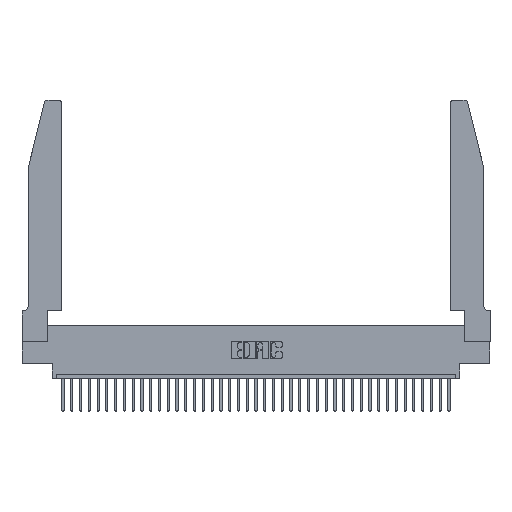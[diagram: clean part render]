
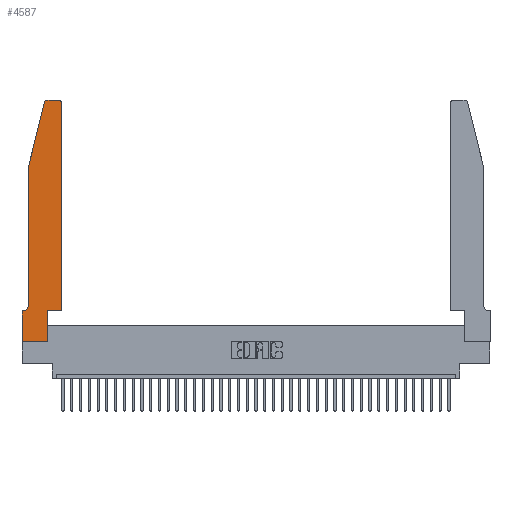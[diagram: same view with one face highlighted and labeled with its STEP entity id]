
A CAD part, top view. The second image highlights one B-rep face of the part: STEP entity #4587.
In plain terms, the highlighted planar face has unit normal (0, 0, 1).
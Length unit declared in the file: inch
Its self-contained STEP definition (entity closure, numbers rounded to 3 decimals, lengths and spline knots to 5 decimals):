
#349 = CARTESIAN_POINT ( 'NONE',  ( 0.284, 2.72, 0.37 ) ) ;
#1829 = AXIS2_PLACEMENT_3D ( 'NONE', #28005, #34072, #10790 ) ;
#2584 = DIRECTION ( 'NONE',  ( 0., 0., 1. ) ) ;
#2587 = AXIS2_PLACEMENT_3D ( 'NONE', #349, #32622, #20655 ) ;
#2610 = CARTESIAN_POINT ( 'NONE',  ( 0.4505, 0.35, 0.37 ) ) ;
#2931 = ORIENTED_EDGE ( 'NONE', *, *, #11599, .T. ) ;
#3148 = VERTEX_POINT ( 'NONE', #26286 ) ;
#3815 = CARTESIAN_POINT ( 'NONE',  ( 0.2605, 2.75, 0.37 ) ) ;
#3861 = VERTEX_POINT ( 'NONE', #38394 ) ;
#3987 = ORIENTED_EDGE ( 'NONE', *, *, #11233, .T. ) ;
#4587 = ADVANCED_FACE ( 'NONE', ( #34450 ), #5657, .T. ) ;
#5254 = VERTEX_POINT ( 'NONE', #12108 ) ;
#5286 = LINE ( 'NONE', #33434, #21419 ) ;
#5390 = VECTOR ( 'NONE', #28375, 39.37008 ) ;
#5592 = ORIENTED_EDGE ( 'NONE', *, *, #9082, .T. ) ;
#5632 = LINE ( 'NONE', #29682, #36201 ) ;
#5657 = PLANE ( 'NONE',  #11920 ) ;
#6202 = CARTESIAN_POINT ( 'NONE',  ( 0.0755, 2., 0.37 ) ) ;
#6476 = ORIENTED_EDGE ( 'NONE', *, *, #26003, .T. ) ;
#6586 = VERTEX_POINT ( 'NONE', #23347 ) ;
#6884 = LINE ( 'NONE', #3815, #20705 ) ;
#7214 = EDGE_CURVE ( 'NONE', #27901, #21540, #31551, .T. ) ;
#7586 = DIRECTION ( 'NONE',  ( -1., 0., 0. ) ) ;
#7918 = VERTEX_POINT ( 'NONE', #31923 ) ;
#8364 = VECTOR ( 'NONE', #17215, 39.37008 ) ;
#8912 = DIRECTION ( 'NONE',  ( 0., -1., 0. ) ) ;
#9082 = EDGE_CURVE ( 'NONE', #3148, #5254, #19011, .T. ) ;
#9666 = DIRECTION ( 'NONE',  ( -1., 0., 0. ) ) ;
#10065 = ORIENTED_EDGE ( 'NONE', *, *, #32586, .T. ) ;
#10258 = VECTOR ( 'NONE', #7586, 39.37008 ) ;
#10413 = CARTESIAN_POINT ( 'NONE',  ( 0.2865, 0.35, 0.37 ) ) ;
#10426 = CARTESIAN_POINT ( 'NONE',  ( 0.0055, 0.42, 0.37 ) ) ;
#10494 = EDGE_CURVE ( 'NONE', #28862, #7918, #6884, .T. ) ;
#10572 = CIRCLE ( 'NONE', #1829, 0.03 ) ;
#10790 = DIRECTION ( 'NONE',  ( 1., 0., 0. ) ) ;
#11145 = CARTESIAN_POINT ( 'NONE',  ( 0., 0., 0.37 ) ) ;
#11233 = EDGE_CURVE ( 'NONE', #3861, #28862, #10572, .T. ) ;
#11424 = CIRCLE ( 'NONE', #26181, 0.07 ) ;
#11599 = EDGE_CURVE ( 'NONE', #33076, #17608, #17524, .T. ) ;
#11644 = ORIENTED_EDGE ( 'NONE', *, *, #7214, .T. ) ;
#11920 = AXIS2_PLACEMENT_3D ( 'NONE', #12030, #2584, #14602 ) ;
#12030 = CARTESIAN_POINT ( 'NONE',  ( 0., 0.35, 0.37 ) ) ;
#12108 = CARTESIAN_POINT ( 'NONE',  ( 0., 0.35, 0.37 ) ) ;
#12353 = LINE ( 'NONE', #10413, #5390 ) ;
#12539 = CARTESIAN_POINT ( 'NONE',  ( 0.4205, 2.75, 0.37 ) ) ;
#12854 = VECTOR ( 'NONE', #28530, 39.37008 ) ;
#12939 = ORIENTED_EDGE ( 'NONE', *, *, #27877, .T. ) ;
#13609 = EDGE_CURVE ( 'NONE', #21540, #3861, #5286, .T. ) ;
#14602 = DIRECTION ( 'NONE',  ( 1., 0., 0. ) ) ;
#15406 = CARTESIAN_POINT ( 'NONE',  ( 0.25487, 2.72718, 0.37 ) ) ;
#15478 = LINE ( 'NONE', #11145, #28899 ) ;
#15664 = CARTESIAN_POINT ( 'NONE',  ( 0.0755, 2., 0.37 ) ) ;
#16342 = DIRECTION ( 'NONE',  ( -1., 0., 0. ) ) ;
#17202 = CARTESIAN_POINT ( 'NONE',  ( 0.2865, 0.35, 0.37 ) ) ;
#17215 = DIRECTION ( 'NONE',  ( 1., 0., 0. ) ) ;
#17524 = LINE ( 'NONE', #30854, #12854 ) ;
#17608 = VERTEX_POINT ( 'NONE', #25983 ) ;
#18871 = EDGE_CURVE ( 'NONE', #36599, #18937, #5632, .T. ) ;
#18937 = VERTEX_POINT ( 'NONE', #15664 ) ;
#19011 = LINE ( 'NONE', #25293, #10258 ) ;
#19884 = DIRECTION ( 'NONE',  ( 0., -1., 0. ) ) ;
#20482 = CIRCLE ( 'NONE', #2587, 0.03 ) ;
#20655 = DIRECTION ( 'NONE',  ( 1., 0., 0. ) ) ;
#20705 = VECTOR ( 'NONE', #9666, 39.37008 ) ;
#20782 = ORIENTED_EDGE ( 'NONE', *, *, #10494, .T. ) ;
#21419 = VECTOR ( 'NONE', #36420, 39.37008 ) ;
#21451 = CARTESIAN_POINT ( 'NONE',  ( 0., 0., 0.37 ) ) ;
#21540 = VERTEX_POINT ( 'NONE', #37667 ) ;
#21776 = EDGE_CURVE ( 'NONE', #6586, #3148, #11424, .T. ) ;
#23347 = CARTESIAN_POINT ( 'NONE',  ( 0.0755, 0.42, 0.37 ) ) ;
#24109 = ORIENTED_EDGE ( 'NONE', *, *, #21776, .T. ) ;
#25293 = CARTESIAN_POINT ( 'NONE',  ( 0.0755, 0.35, 0.37 ) ) ;
#25983 = CARTESIAN_POINT ( 'NONE',  ( 0.2865, 0., 0.37 ) ) ;
#26003 = EDGE_CURVE ( 'NONE', #18937, #6586, #34702, .T. ) ;
#26056 = ORIENTED_EDGE ( 'NONE', *, *, #37195, .T. ) ;
#26181 = AXIS2_PLACEMENT_3D ( 'NONE', #10426, #31137, #16342 ) ;
#26217 = EDGE_LOOP ( 'NONE', ( #20782, #26056, #30105, #6476, #24109, #5592, #12939, #2931, #10065, #11644, #27728, #3987 ) ) ;
#26286 = CARTESIAN_POINT ( 'NONE',  ( 0.0055, 0.35, 0.37 ) ) ;
#27728 = ORIENTED_EDGE ( 'NONE', *, *, #13609, .T. ) ;
#27877 = EDGE_CURVE ( 'NONE', #5254, #33076, #15478, .T. ) ;
#27901 = VERTEX_POINT ( 'NONE', #17202 ) ;
#28005 = CARTESIAN_POINT ( 'NONE',  ( 0.4205, 2.72, 0.37 ) ) ;
#28375 = DIRECTION ( 'NONE',  ( 0., 1., 0. ) ) ;
#28530 = DIRECTION ( 'NONE',  ( 1., 0., 0. ) ) ;
#28862 = VERTEX_POINT ( 'NONE', #12539 ) ;
#28899 = VECTOR ( 'NONE', #19884, 39.37008 ) ;
#29682 = CARTESIAN_POINT ( 'NONE',  ( 0.0755, 2., 0.37 ) ) ;
#30105 = ORIENTED_EDGE ( 'NONE', *, *, #18871, .T. ) ;
#30854 = CARTESIAN_POINT ( 'NONE',  ( 0., 0., 0.37 ) ) ;
#31137 = DIRECTION ( 'NONE',  ( 0., 0., -1. ) ) ;
#31551 = LINE ( 'NONE', #2610, #8364 ) ;
#31923 = CARTESIAN_POINT ( 'NONE',  ( 0.284, 2.75, 0.37 ) ) ;
#32586 = EDGE_CURVE ( 'NONE', #17608, #27901, #12353, .T. ) ;
#32622 = DIRECTION ( 'NONE',  ( 0., 0., 1. ) ) ;
#32651 = DIRECTION ( 'NONE',  ( -0.239, -0.971, 0. ) ) ;
#33076 = VERTEX_POINT ( 'NONE', #21451 ) ;
#33434 = CARTESIAN_POINT ( 'NONE',  ( 0.4505, 0.35, 0.37 ) ) ;
#34072 = DIRECTION ( 'NONE',  ( 0., 0., 1. ) ) ;
#34253 = VECTOR ( 'NONE', #8912, 39.37008 ) ;
#34450 = FACE_OUTER_BOUND ( 'NONE', #26217, .T. ) ;
#34702 = LINE ( 'NONE', #6202, #34253 ) ;
#36201 = VECTOR ( 'NONE', #32651, 39.37008 ) ;
#36420 = DIRECTION ( 'NONE',  ( 0., 1., 0. ) ) ;
#36599 = VERTEX_POINT ( 'NONE', #15406 ) ;
#37195 = EDGE_CURVE ( 'NONE', #7918, #36599, #20482, .T. ) ;
#37667 = CARTESIAN_POINT ( 'NONE',  ( 0.4505, 0.35, 0.37 ) ) ;
#38394 = CARTESIAN_POINT ( 'NONE',  ( 0.4505, 2.72, 0.37 ) ) ;
